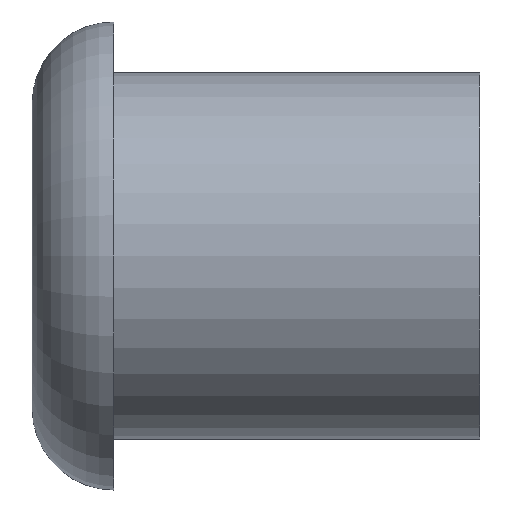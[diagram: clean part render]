
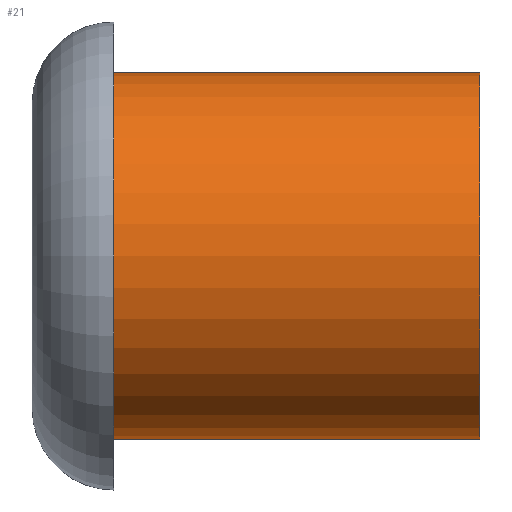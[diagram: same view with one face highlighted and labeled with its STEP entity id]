
A CAD part, left-side view. The second image highlights one B-rep face of the part: STEP entity #21.
In plain terms, the highlighted cylindrical face has radius 4.5 mm (diameter 9 mm), a partial arc.
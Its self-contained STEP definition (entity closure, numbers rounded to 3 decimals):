
#4 = FACE_OUTER_BOUND ( 'NONE', #98, .T. ) ;
#6 = LINE ( 'NONE', #255, #67 ) ;
#21 = ADVANCED_FACE ( 'NONE', ( #4 ), #64, .T. ) ;
#27 = CARTESIAN_POINT ( 'NONE',  ( 0., 0., 0. ) ) ;
#41 = ORIENTED_EDGE ( 'NONE', *, *, #101, .T. ) ;
#42 = DIRECTION ( 'NONE',  ( 0., -1., 0. ) ) ;
#54 = DIRECTION ( 'NONE',  ( 0., 0., 1. ) ) ;
#55 = CARTESIAN_POINT ( 'NONE',  ( 0., 9., -4.5 ) ) ;
#64 = CYLINDRICAL_SURFACE ( 'NONE', #128, 4.5 ) ;
#67 = VECTOR ( 'NONE', #42, 1000. ) ;
#74 = VECTOR ( 'NONE', #212, 1000. ) ;
#96 = DIRECTION ( 'NONE',  ( 0., 1., 0. ) ) ;
#98 = EDGE_LOOP ( 'NONE', ( #149, #204, #269, #41 ) ) ;
#101 = EDGE_CURVE ( 'NONE', #264, #105, #292, .T. ) ;
#105 = VERTEX_POINT ( 'NONE', #173 ) ;
#109 = AXIS2_PLACEMENT_3D ( 'NONE', #220, #96, #247 ) ;
#112 = DIRECTION ( 'NONE',  ( 0., -1., 0. ) ) ;
#126 = AXIS2_PLACEMENT_3D ( 'NONE', #27, #174, #54 ) ;
#128 = AXIS2_PLACEMENT_3D ( 'NONE', #151, #112, #134 ) ;
#134 = DIRECTION ( 'NONE',  ( 0., 0., -1. ) ) ;
#145 = EDGE_CURVE ( 'NONE', #152, #147, #281, .T. ) ;
#147 = VERTEX_POINT ( 'NONE', #296 ) ;
#149 = ORIENTED_EDGE ( 'NONE', *, *, #284, .F. ) ;
#151 = CARTESIAN_POINT ( 'NONE',  ( 0., 9., 0. ) ) ;
#152 = VERTEX_POINT ( 'NONE', #55 ) ;
#173 = CARTESIAN_POINT ( 'NONE',  ( 0., 0., 4.5 ) ) ;
#174 = DIRECTION ( 'NONE',  ( 0., 1., 0. ) ) ;
#183 = LINE ( 'NONE', #188, #74 ) ;
#188 = CARTESIAN_POINT ( 'NONE',  ( 0., 9., 4.5 ) ) ;
#204 = ORIENTED_EDGE ( 'NONE', *, *, #145, .F. ) ;
#208 = CARTESIAN_POINT ( 'NONE',  ( 0., 0., -4.5 ) ) ;
#212 = DIRECTION ( 'NONE',  ( 0., -1., 0. ) ) ;
#220 = CARTESIAN_POINT ( 'NONE',  ( 0., 9., 0. ) ) ;
#247 = DIRECTION ( 'NONE',  ( 0., 0., 1. ) ) ;
#255 = CARTESIAN_POINT ( 'NONE',  ( 0., 9., -4.5 ) ) ;
#264 = VERTEX_POINT ( 'NONE', #208 ) ;
#269 = ORIENTED_EDGE ( 'NONE', *, *, #282, .T. ) ;
#281 = CIRCLE ( 'NONE', #109, 4.5 ) ;
#282 = EDGE_CURVE ( 'NONE', #152, #264, #6, .T. ) ;
#284 = EDGE_CURVE ( 'NONE', #147, #105, #183, .T. ) ;
#292 = CIRCLE ( 'NONE', #126, 4.5 ) ;
#296 = CARTESIAN_POINT ( 'NONE',  ( 0., 9., 4.5 ) ) ;
